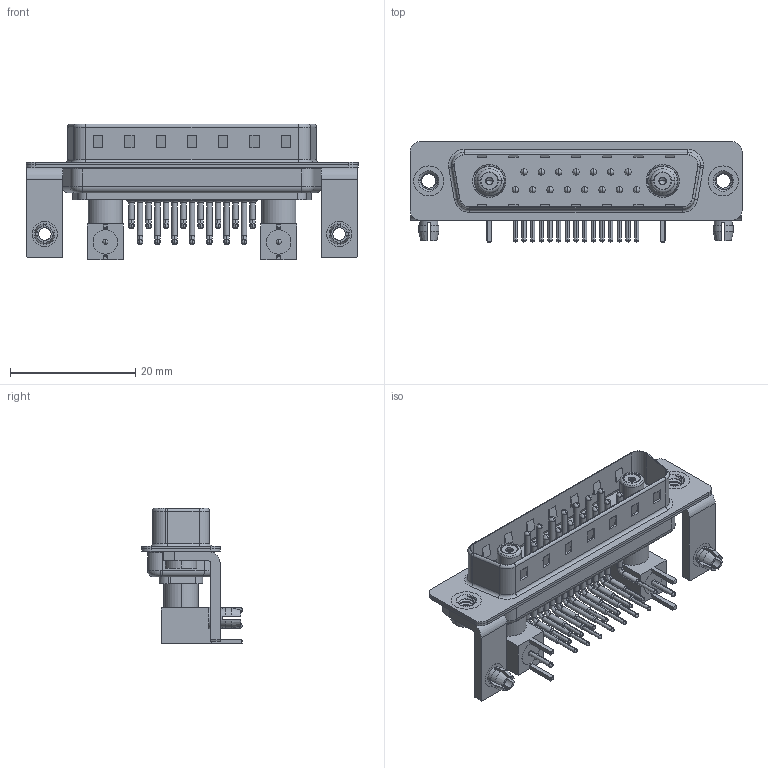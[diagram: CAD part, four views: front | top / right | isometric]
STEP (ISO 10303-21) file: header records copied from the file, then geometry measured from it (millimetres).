
FILE_DESCRIPTION (( 'STEP AP203' ), '1' );
FILE_NAME ('629-17W2640-5NB.STEP', '2022-05-10T16:24:29', ( '' ), ( '' ), 'SwSTEP 2.0', 'SolidWorks 2020', '' );
FILE_SCHEMA (( 'CONFIG_CONTROL_DESIGN' ));
Length unit declared in the file: millimetre
Products named in the file (18): 629Combo Board Lock; 629Combo Shell Rear_25 Contacts; Co-Ax Jack Assy_RA; 629-17W2640-5NB; 629Combo Housing_17W2; 629Combo Contact Row 1; Socket_RA; 629Combo Stabilizer Bracket; Insulator Socket 2; Locking Collar; Co-Ax Jack_RA PC Tail; Insulator RA Pin; Insulator Socket; 629Combo Threaded Rivet_2; 629Combo Contact Row 2; RA Back Shell; 629Combo Shell Front_25 Contacts
Assembly tree (40 placements, depth 3):
  629-17W2640-5NB
    629Combo Housing_17W2
    629Combo Shell Rear_25 Contacts
    629Combo Shell Front_25 Contacts
    629Combo Threaded Rivet_2  x2
    629Combo Stabilizer Bracket  x2
    629Combo Board Lock  x2
    Co-Ax Jack Assy_RA
      Co-Ax Jack_RA PC Tail
      Insulator Socket
      Insulator Socket 2
      Locking Collar
      Socket_RA
      RA Back Shell
      Insulator RA Pin
    Co-Ax Jack Assy_RA
      Co-Ax Jack_RA PC Tail
      Insulator Socket
      Insulator Socket 2
      Locking Collar
      Socket_RA
      RA Back Shell
      Insulator RA Pin
    629Combo Contact Row 1  x7
    629Combo Contact Row 2  x8
Bounding box: 53.05 x 16 x 21.71 mm (x, y, z)
Volume: 3756.9 mm3; surface area: 10017.2 mm2
Topology: 38 solids, 38 shells, 2470 faces, 6683 edges, 4316 vertices
Faces by surface type: plane 1313, cylinder 867, cone 126, bspline 98, torus 62, sphere 4
Entity records: 31493 total; most frequent: CARTESIAN_POINT 6605, DIRECTION 4894, ORIENTED_EDGE 4510, EDGE_CURVE 2255, AXIS2_PLACEMENT_3D 1789, VERTEX_POINT 1453, VECTOR 1316, LINE 1316
